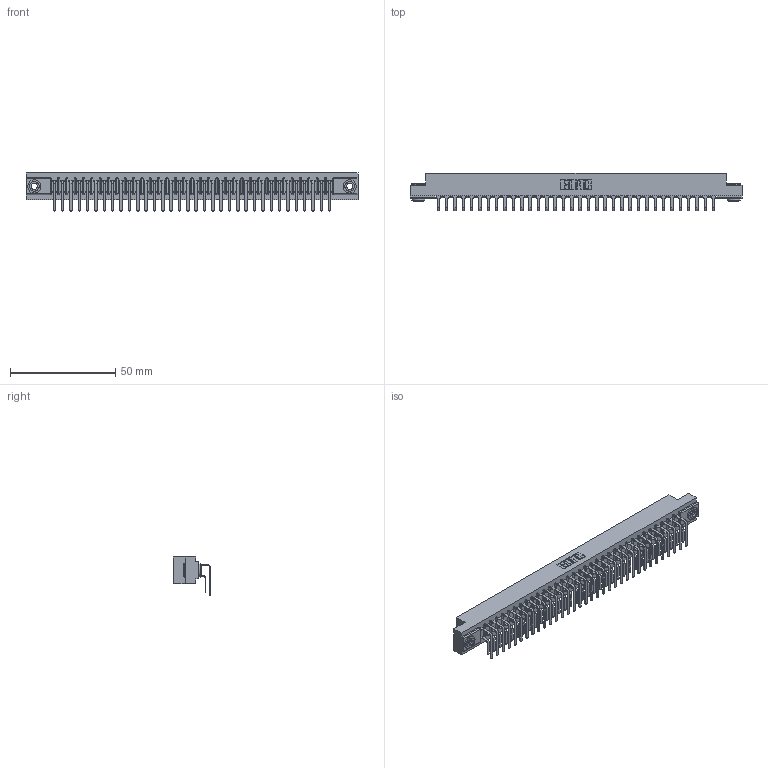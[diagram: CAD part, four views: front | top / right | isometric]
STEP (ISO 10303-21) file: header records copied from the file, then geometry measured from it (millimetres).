
FILE_DESCRIPTION (( 'STEP AP203' ), '1' );
FILE_NAME ('357-068-559-203.STEP', '2018-08-12T18:22:25', ( '' ), ( '' ), 'SwSTEP 2.0', 'SolidWorks 2016', '' );
FILE_SCHEMA (( 'CONFIG_CONTROL_DESIGN' ));
Length unit declared in the file: inch
Products named in the file (5): 307-290-001_559 - 2 (Single); 345-250-002_345-250-002-102; 357-068-559-203; 307 Part_.156 Dia Mounting Holes; 307-290-001_558 559 - 1 (Single)
Assembly tree (71 placements, depth 2):
  357-068-559-203
    307 Part_.156 Dia Mounting Holes
    307-290-001_558 559 - 1 (Single)  x34
    307-290-001_559 - 2 (Single)  x34
    345-250-002_345-250-002-102  x2
Bounding box: 157.73 x 17.69 x 18.07 mm (x, y, z)
Volume: 17019.2 mm3; surface area: 22669.2 mm2
Topology: 71 solids, 71 shells, 3605 faces, 10091 edges, 6538 vertices
Faces by surface type: plane 2338, cylinder 1189, sphere 70, cone 8
Entity records: 33734 total; most frequent: CARTESIAN_POINT 5505, ORIENTED_EDGE 5446, DIRECTION 5409, EDGE_CURVE 2723, VECTOR 2077, LINE 2077, VERTEX_POINT 1762, AXIS2_PLACEMENT_3D 1666
